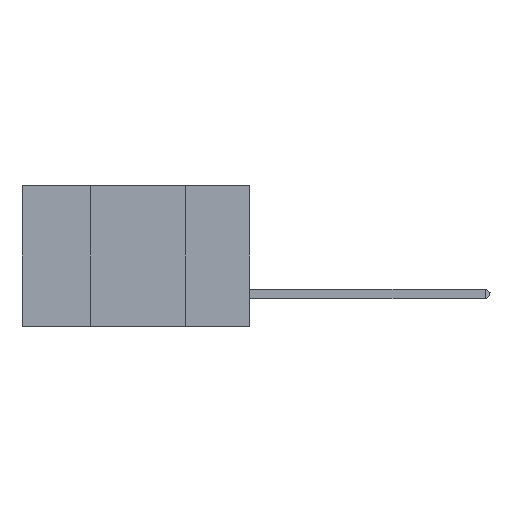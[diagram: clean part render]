
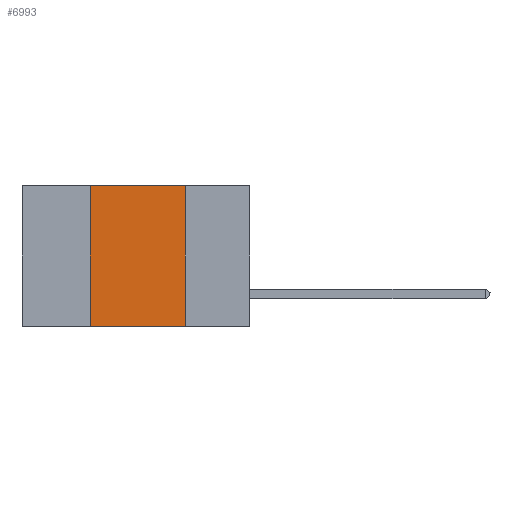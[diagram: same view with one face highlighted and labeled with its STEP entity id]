
A CAD part, left-side view. The second image highlights one B-rep face of the part: STEP entity #6993.
In plain terms, the highlighted planar face has unit normal (-1, 0, 0).
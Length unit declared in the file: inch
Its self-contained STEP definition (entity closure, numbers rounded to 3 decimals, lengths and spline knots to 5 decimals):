
#3502 = LINE ( 'NONE', #37975, #25213 ) ;
#4787 = VERTEX_POINT ( 'NONE', #25190 ) ;
#5035 = DIRECTION ( 'NONE',  ( 0., -1., 0. ) ) ;
#5505 = DIRECTION ( 'NONE',  ( 0., 0., -1. ) ) ;
#6002 = EDGE_CURVE ( 'NONE', #4787, #15449, #36036, .T. ) ;
#6188 = CARTESIAN_POINT ( 'NONE',  ( 0., 0.17, -0.37 ) ) ;
#6993 = ADVANCED_FACE ( 'NONE', ( #22940 ), #12067, .F. ) ;
#10160 = VECTOR ( 'NONE', #20988, 39.37008 ) ;
#12067 = PLANE ( 'NONE',  #15156 ) ;
#12315 = VERTEX_POINT ( 'NONE', #6188 ) ;
#13953 = EDGE_CURVE ( 'NONE', #4787, #12315, #24087, .T. ) ;
#15117 = CARTESIAN_POINT ( 'NONE',  ( 0., 0.42, 0. ) ) ;
#15156 = AXIS2_PLACEMENT_3D ( 'NONE', #18358, #25299, #21690 ) ;
#15449 = VERTEX_POINT ( 'NONE', #19066 ) ;
#16895 = VECTOR ( 'NONE', #5035, 39.37008 ) ;
#18039 = CARTESIAN_POINT ( 'NONE',  ( 0., 0.17, 0. ) ) ;
#18358 = CARTESIAN_POINT ( 'NONE',  ( 0., 0.6, 0. ) ) ;
#18725 = CARTESIAN_POINT ( 'NONE',  ( 0., 0.6, -0.37 ) ) ;
#19066 = CARTESIAN_POINT ( 'NONE',  ( 0., 0.42, 0. ) ) ;
#19151 = EDGE_CURVE ( 'NONE', #15449, #24926, #26634, .T. ) ;
#20252 = CARTESIAN_POINT ( 'NONE',  ( 0., 0.6, 0. ) ) ;
#20551 = ORIENTED_EDGE ( 'NONE', *, *, #19151, .F. ) ;
#20988 = DIRECTION ( 'NONE',  ( 0., -1., 0. ) ) ;
#21690 = DIRECTION ( 'NONE',  ( 0., 0., -1. ) ) ;
#22940 = FACE_OUTER_BOUND ( 'NONE', #38046, .T. ) ;
#24023 = ORIENTED_EDGE ( 'NONE', *, *, #13953, .T. ) ;
#24087 = LINE ( 'NONE', #18725, #16895 ) ;
#24926 = VERTEX_POINT ( 'NONE', #18039 ) ;
#25190 = CARTESIAN_POINT ( 'NONE',  ( 0., 0.42, -0.37 ) ) ;
#25213 = VECTOR ( 'NONE', #5505, 39.37008 ) ;
#25299 = DIRECTION ( 'NONE',  ( 1., 0., 0. ) ) ;
#26634 = LINE ( 'NONE', #20252, #10160 ) ;
#27123 = VECTOR ( 'NONE', #31781, 39.37008 ) ;
#30689 = EDGE_CURVE ( 'NONE', #24926, #12315, #3502, .T. ) ;
#31781 = DIRECTION ( 'NONE',  ( 0., 0., 1. ) ) ;
#36036 = LINE ( 'NONE', #15117, #27123 ) ;
#36587 = ORIENTED_EDGE ( 'NONE', *, *, #30689, .F. ) ;
#37331 = ORIENTED_EDGE ( 'NONE', *, *, #6002, .F. ) ;
#37975 = CARTESIAN_POINT ( 'NONE',  ( 0., 0.17, 0. ) ) ;
#38046 = EDGE_LOOP ( 'NONE', ( #36587, #20551, #37331, #24023 ) ) ;
